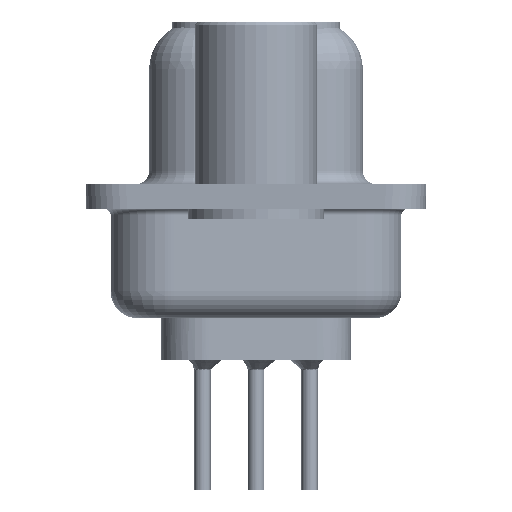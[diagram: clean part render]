
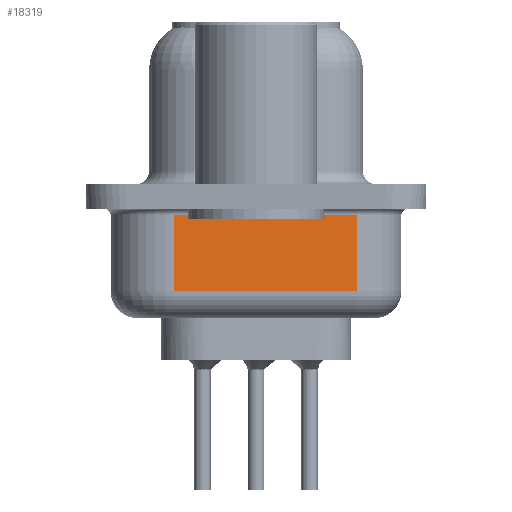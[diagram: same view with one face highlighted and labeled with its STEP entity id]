
A CAD part, left-side view. The second image highlights one B-rep face of the part: STEP entity #18319.
In plain terms, the highlighted planar face has unit normal (-0.985, -0.174, 0).
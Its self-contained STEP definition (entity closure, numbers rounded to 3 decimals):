
#634 = LINE ( 'NONE', #8789, #8049 ) ;
#1126 = EDGE_CURVE ( 'NONE', #11165, #22857, #634, .T. ) ;
#1248 = ORIENTED_EDGE ( 'NONE', *, *, #31371, .F. ) ;
#1381 = CARTESIAN_POINT ( 'NONE',  ( 4.031, -3.722, -0.7 ) ) ;
#2010 = VERTEX_POINT ( 'NONE', #3119 ) ;
#3119 = CARTESIAN_POINT ( 'NONE',  ( 2.84, 3.028, -0.7 ) ) ;
#3187 = VECTOR ( 'NONE', #6540, 1000. ) ;
#4536 = CARTESIAN_POINT ( 'NONE',  ( 2.84, 3.028, -4.5 ) ) ;
#4649 = PLANE ( 'NONE',  #20143 ) ;
#6381 = VECTOR ( 'NONE', #21636, 1000. ) ;
#6540 = DIRECTION ( 'NONE',  ( 0., 0., 1. ) ) ;
#6866 = CARTESIAN_POINT ( 'NONE',  ( 2.84, 3.028, -3.5 ) ) ;
#8049 = VECTOR ( 'NONE', #16102, 1000. ) ;
#8409 = ORIENTED_EDGE ( 'NONE', *, *, #32176, .T. ) ;
#8789 = CARTESIAN_POINT ( 'NONE',  ( 2.84, 3.028, -3.5 ) ) ;
#10415 = VERTEX_POINT ( 'NONE', #1381 ) ;
#11165 = VERTEX_POINT ( 'NONE', #6866 ) ;
#11254 = CARTESIAN_POINT ( 'NONE',  ( 2.84, 3.028, -0.7 ) ) ;
#13075 = ORIENTED_EDGE ( 'NONE', *, *, #1126, .T. ) ;
#15178 = DIRECTION ( 'NONE',  ( 0.985, 0.174, 0. ) ) ;
#16102 = DIRECTION ( 'NONE',  ( 0.174, -0.985, 0. ) ) ;
#17716 = CARTESIAN_POINT ( 'NONE',  ( 2.84, 3.028, -4.5 ) ) ;
#18093 = EDGE_LOOP ( 'NONE', ( #1248, #13075, #23674, #8409 ) ) ;
#18319 = ADVANCED_FACE ( 'NONE', ( #20108 ), #4649, .F. ) ;
#19291 = CARTESIAN_POINT ( 'NONE',  ( 4.031, -3.722, -4.5 ) ) ;
#20108 = FACE_OUTER_BOUND ( 'NONE', #18093, .T. ) ;
#20143 = AXIS2_PLACEMENT_3D ( 'NONE', #17716, #15178, #22832 ) ;
#20636 = CARTESIAN_POINT ( 'NONE',  ( 4.031, -3.722, -3.5 ) ) ;
#21636 = DIRECTION ( 'NONE',  ( -0.174, 0.985, 0. ) ) ;
#22832 = DIRECTION ( 'NONE',  ( -0.174, 0.985, 0. ) ) ;
#22857 = VERTEX_POINT ( 'NONE', #20636 ) ;
#23674 = ORIENTED_EDGE ( 'NONE', *, *, #31857, .T. ) ;
#27836 = DIRECTION ( 'NONE',  ( 0., 0., 1. ) ) ;
#29489 = LINE ( 'NONE', #11254, #6381 ) ;
#29689 = LINE ( 'NONE', #19291, #3187 ) ;
#30876 = VECTOR ( 'NONE', #27836, 1000. ) ;
#31371 = EDGE_CURVE ( 'NONE', #11165, #2010, #32604, .T. ) ;
#31857 = EDGE_CURVE ( 'NONE', #22857, #10415, #29689, .T. ) ;
#32176 = EDGE_CURVE ( 'NONE', #10415, #2010, #29489, .T. ) ;
#32604 = LINE ( 'NONE', #4536, #30876 ) ;
